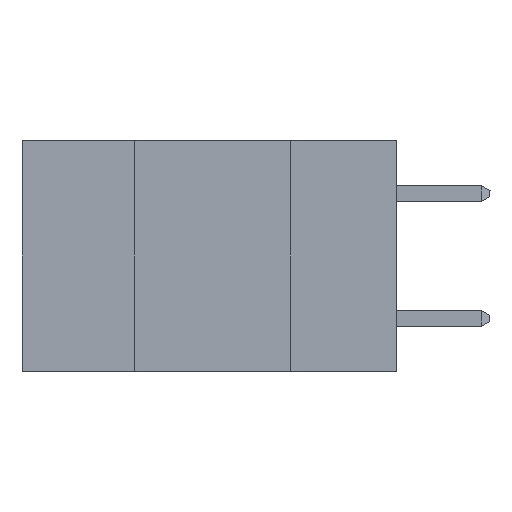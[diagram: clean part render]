
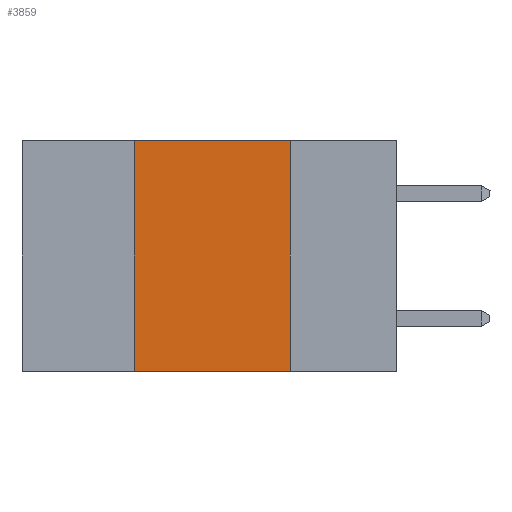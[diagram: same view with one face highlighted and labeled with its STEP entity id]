
A CAD part, left-side view. The second image highlights one B-rep face of the part: STEP entity #3859.
In plain terms, the highlighted planar face has unit normal (-1, 0, 0).
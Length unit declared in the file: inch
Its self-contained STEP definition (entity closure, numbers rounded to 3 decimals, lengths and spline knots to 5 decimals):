
#759 = VERTEX_POINT ( 'NONE', #14513 ) ;
#1145 = VERTEX_POINT ( 'NONE', #13900 ) ;
#1293 = LINE ( 'NONE', #14086, #17267 ) ;
#1788 = ORIENTED_EDGE ( 'NONE', *, *, #18200, .T. ) ;
#2276 = CARTESIAN_POINT ( 'NONE',  ( 0., 0.42, 0. ) ) ;
#2465 = DIRECTION ( 'NONE',  ( 0., 0., 1. ) ) ;
#2823 = LINE ( 'NONE', #16276, #13746 ) ;
#3432 = EDGE_CURVE ( 'NONE', #3765, #759, #16470, .T. ) ;
#3765 = VERTEX_POINT ( 'NONE', #10947 ) ;
#3859 = ADVANCED_FACE ( 'NONE', ( #17384 ), #11061, .F. ) ;
#5697 = DIRECTION ( 'NONE',  ( 0., -1., 0. ) ) ;
#5713 = CARTESIAN_POINT ( 'NONE',  ( 0., 0.6, 0. ) ) ;
#8467 = ORIENTED_EDGE ( 'NONE', *, *, #3432, .F. ) ;
#8801 = DIRECTION ( 'NONE',  ( 0., 0., -1. ) ) ;
#8840 = DIRECTION ( 'NONE',  ( 1., 0., 0. ) ) ;
#8868 = CARTESIAN_POINT ( 'NONE',  ( 0., 0.6, 0. ) ) ;
#9135 = EDGE_CURVE ( 'NONE', #759, #1145, #16740, .T. ) ;
#9775 = CARTESIAN_POINT ( 'NONE',  ( 0., 0.17, -0.37 ) ) ;
#10197 = DIRECTION ( 'NONE',  ( 0., -1., 0. ) ) ;
#10368 = ORIENTED_EDGE ( 'NONE', *, *, #9135, .F. ) ;
#10947 = CARTESIAN_POINT ( 'NONE',  ( 0., 0.42, -0.37 ) ) ;
#11061 = PLANE ( 'NONE',  #16374 ) ;
#11902 = ORIENTED_EDGE ( 'NONE', *, *, #13122, .F. ) ;
#12382 = VECTOR ( 'NONE', #2465, 39.37008 ) ;
#12508 = EDGE_LOOP ( 'NONE', ( #11902, #10368, #8467, #1788 ) ) ;
#13113 = VECTOR ( 'NONE', #5697, 39.37008 ) ;
#13122 = EDGE_CURVE ( 'NONE', #1145, #13228, #1293, .T. ) ;
#13228 = VERTEX_POINT ( 'NONE', #9775 ) ;
#13746 = VECTOR ( 'NONE', #10197, 39.37008 ) ;
#13900 = CARTESIAN_POINT ( 'NONE',  ( 0., 0.17, 0. ) ) ;
#14086 = CARTESIAN_POINT ( 'NONE',  ( 0., 0.17, 0. ) ) ;
#14513 = CARTESIAN_POINT ( 'NONE',  ( 0., 0.42, 0. ) ) ;
#16276 = CARTESIAN_POINT ( 'NONE',  ( 0., 0.6, -0.37 ) ) ;
#16374 = AXIS2_PLACEMENT_3D ( 'NONE', #8868, #8840, #8801 ) ;
#16470 = LINE ( 'NONE', #2276, #12382 ) ;
#16740 = LINE ( 'NONE', #5713, #13113 ) ;
#17221 = DIRECTION ( 'NONE',  ( 0., 0., -1. ) ) ;
#17267 = VECTOR ( 'NONE', #17221, 39.37008 ) ;
#17384 = FACE_OUTER_BOUND ( 'NONE', #12508, .T. ) ;
#18200 = EDGE_CURVE ( 'NONE', #3765, #13228, #2823, .T. ) ;
